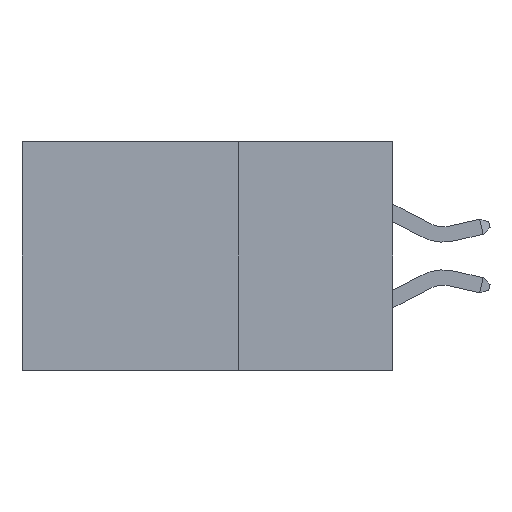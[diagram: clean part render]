
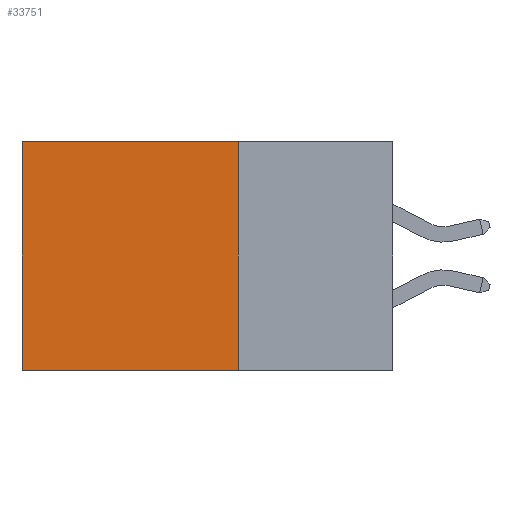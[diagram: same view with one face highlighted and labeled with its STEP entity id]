
A CAD part, left-side view. The second image highlights one B-rep face of the part: STEP entity #33751.
In plain terms, the highlighted planar face has unit normal (-1, 0, 0).
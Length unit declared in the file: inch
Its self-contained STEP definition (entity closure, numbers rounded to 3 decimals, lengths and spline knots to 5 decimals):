
#258 = ORIENTED_EDGE ( 'NONE', *, *, #36016, .F. ) ;
#1376 = VECTOR ( 'NONE', #36417, 39.37008 ) ;
#2751 = VECTOR ( 'NONE', #22724, 39.37008 ) ;
#3148 = EDGE_CURVE ( 'NONE', #33173, #18680, #29729, .T. ) ;
#4055 = EDGE_CURVE ( 'NONE', #26054, #33173, #34700, .T. ) ;
#8016 = VERTEX_POINT ( 'NONE', #33114 ) ;
#8535 = EDGE_LOOP ( 'NONE', ( #26798, #258, #40355, #9674 ) ) ;
#9674 = ORIENTED_EDGE ( 'NONE', *, *, #4055, .T. ) ;
#11929 = EDGE_CURVE ( 'NONE', #26054, #8016, #36499, .T. ) ;
#13753 = DIRECTION ( 'NONE',  ( 0., 1., 0. ) ) ;
#14127 = CARTESIAN_POINT ( 'NONE',  ( 0.2875, 0.25, 0. ) ) ;
#14772 = VECTOR ( 'NONE', #37293, 39.37008 ) ;
#15332 = LINE ( 'NONE', #16333, #2751 ) ;
#15389 = CARTESIAN_POINT ( 'NONE',  ( 0.2875, 0.25, 0. ) ) ;
#16333 = CARTESIAN_POINT ( 'NONE',  ( 0.2875, 0.25, -0.37 ) ) ;
#17344 = PLANE ( 'NONE',  #26231 ) ;
#18680 = VERTEX_POINT ( 'NONE', #22198 ) ;
#20521 = DIRECTION ( 'NONE',  ( 1., 0., 0. ) ) ;
#20728 = CARTESIAN_POINT ( 'NONE',  ( 0.2875, 0.25, 0. ) ) ;
#22198 = CARTESIAN_POINT ( 'NONE',  ( 0.2875, 0.6, -0.37 ) ) ;
#22724 = DIRECTION ( 'NONE',  ( 0., 1., 0. ) ) ;
#26054 = VERTEX_POINT ( 'NONE', #27916 ) ;
#26231 = AXIS2_PLACEMENT_3D ( 'NONE', #14127, #20521, #39766 ) ;
#26798 = ORIENTED_EDGE ( 'NONE', *, *, #3148, .T. ) ;
#27916 = CARTESIAN_POINT ( 'NONE',  ( 0.2875, 0.25, 0. ) ) ;
#29729 = LINE ( 'NONE', #36704, #14772 ) ;
#33114 = CARTESIAN_POINT ( 'NONE',  ( 0.2875, 0.25, -0.37 ) ) ;
#33173 = VERTEX_POINT ( 'NONE', #36987 ) ;
#33697 = VECTOR ( 'NONE', #13753, 39.37008 ) ;
#33751 = ADVANCED_FACE ( 'NONE', ( #37109 ), #17344, .F. ) ;
#34700 = LINE ( 'NONE', #15389, #33697 ) ;
#36016 = EDGE_CURVE ( 'NONE', #8016, #18680, #15332, .T. ) ;
#36417 = DIRECTION ( 'NONE',  ( 0., 0., -1. ) ) ;
#36499 = LINE ( 'NONE', #20728, #1376 ) ;
#36704 = CARTESIAN_POINT ( 'NONE',  ( 0.2875, 0.6, 0. ) ) ;
#36987 = CARTESIAN_POINT ( 'NONE',  ( 0.2875, 0.6, 0. ) ) ;
#37109 = FACE_OUTER_BOUND ( 'NONE', #8535, .T. ) ;
#37293 = DIRECTION ( 'NONE',  ( 0., 0., -1. ) ) ;
#39766 = DIRECTION ( 'NONE',  ( 0., 0., -1. ) ) ;
#40355 = ORIENTED_EDGE ( 'NONE', *, *, #11929, .F. ) ;
